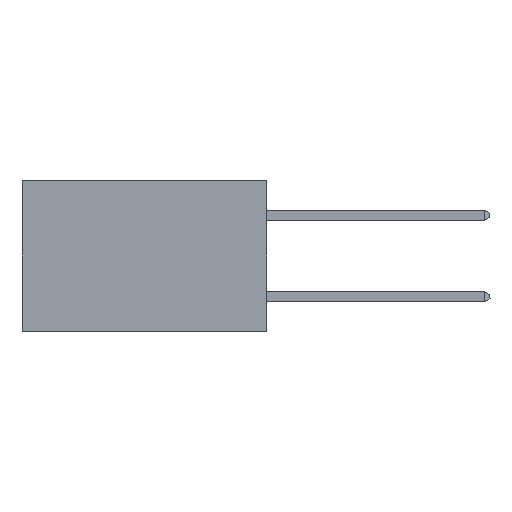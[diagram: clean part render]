
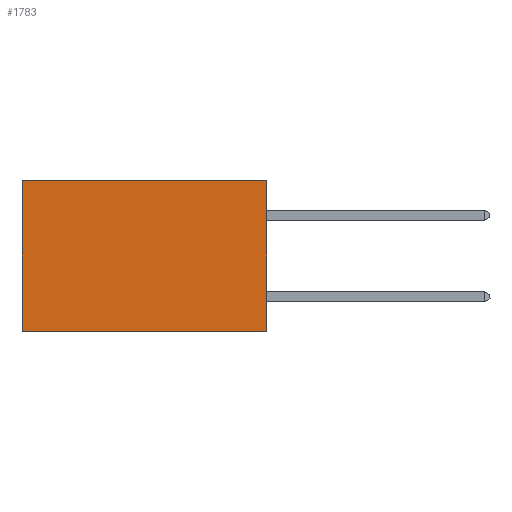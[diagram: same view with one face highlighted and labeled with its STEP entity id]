
A CAD part, left-side view. The second image highlights one B-rep face of the part: STEP entity #1783.
In plain terms, the highlighted planar face has unit normal (-1, 0, 0).
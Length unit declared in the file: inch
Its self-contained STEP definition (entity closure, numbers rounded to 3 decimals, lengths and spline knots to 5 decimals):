
#161 = AXIS2_PLACEMENT_3D ( 'NONE', #3058, #11961, #5286 ) ;
#282 = VECTOR ( 'NONE', #13731, 39.37008 ) ;
#409 = DIRECTION ( 'NONE',  ( 0., 1., 0. ) ) ;
#930 = DIRECTION ( 'NONE',  ( 0., 0., -1. ) ) ;
#1187 = CARTESIAN_POINT ( 'NONE',  ( 0.2875, 0.6, 0. ) ) ;
#1783 = ADVANCED_FACE ( 'NONE', ( #12433 ), #9695, .F. ) ;
#2001 = DIRECTION ( 'NONE',  ( 0., 0., -1. ) ) ;
#2355 = CARTESIAN_POINT ( 'NONE',  ( 0.2875, 0., 0. ) ) ;
#2605 = EDGE_LOOP ( 'NONE', ( #7150, #3317, #9363, #2677 ) ) ;
#2677 = ORIENTED_EDGE ( 'NONE', *, *, #11402, .T. ) ;
#3058 = CARTESIAN_POINT ( 'NONE',  ( 0.2875, 0., 0. ) ) ;
#3317 = ORIENTED_EDGE ( 'NONE', *, *, #8531, .F. ) ;
#3958 = LINE ( 'NONE', #7200, #6791 ) ;
#4426 = CARTESIAN_POINT ( 'NONE',  ( 0.2875, 0.6, -0.37 ) ) ;
#5069 = LINE ( 'NONE', #2355, #282 ) ;
#5286 = DIRECTION ( 'NONE',  ( 0., 0., -1. ) ) ;
#5347 = VERTEX_POINT ( 'NONE', #9929 ) ;
#5394 = EDGE_CURVE ( 'NONE', #7294, #7584, #6696, .T. ) ;
#6696 = LINE ( 'NONE', #7701, #12468 ) ;
#6791 = VECTOR ( 'NONE', #409, 39.37008 ) ;
#7150 = ORIENTED_EDGE ( 'NONE', *, *, #5394, .T. ) ;
#7200 = CARTESIAN_POINT ( 'NONE',  ( 0.2875, 0., -0.37 ) ) ;
#7294 = VERTEX_POINT ( 'NONE', #1187 ) ;
#7584 = VERTEX_POINT ( 'NONE', #4426 ) ;
#7701 = CARTESIAN_POINT ( 'NONE',  ( 0.2875, 0.6, 0. ) ) ;
#7704 = VECTOR ( 'NONE', #2001, 39.37008 ) ;
#8240 = EDGE_CURVE ( 'NONE', #10429, #5347, #12199, .T. ) ;
#8531 = EDGE_CURVE ( 'NONE', #5347, #7584, #3958, .T. ) ;
#8713 = CARTESIAN_POINT ( 'NONE',  ( 0.2875, 0., 0. ) ) ;
#9363 = ORIENTED_EDGE ( 'NONE', *, *, #8240, .F. ) ;
#9695 = PLANE ( 'NONE',  #161 ) ;
#9929 = CARTESIAN_POINT ( 'NONE',  ( 0.2875, 0., -0.37 ) ) ;
#10429 = VERTEX_POINT ( 'NONE', #10560 ) ;
#10560 = CARTESIAN_POINT ( 'NONE',  ( 0.2875, 0., 0. ) ) ;
#11402 = EDGE_CURVE ( 'NONE', #10429, #7294, #5069, .T. ) ;
#11961 = DIRECTION ( 'NONE',  ( 1., 0., 0. ) ) ;
#12199 = LINE ( 'NONE', #8713, #7704 ) ;
#12433 = FACE_OUTER_BOUND ( 'NONE', #2605, .T. ) ;
#12468 = VECTOR ( 'NONE', #930, 39.37008 ) ;
#13731 = DIRECTION ( 'NONE',  ( 0., 1., 0. ) ) ;
